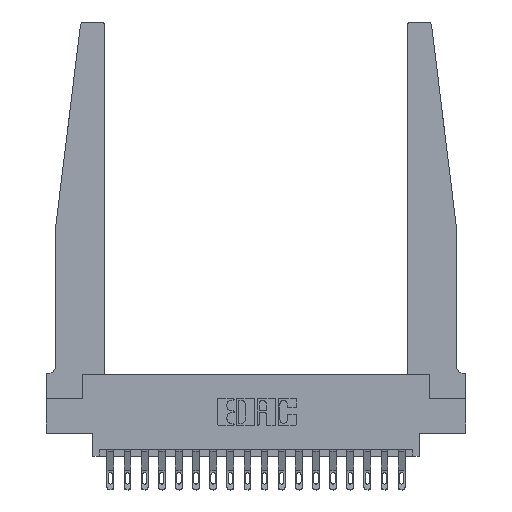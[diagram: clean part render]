
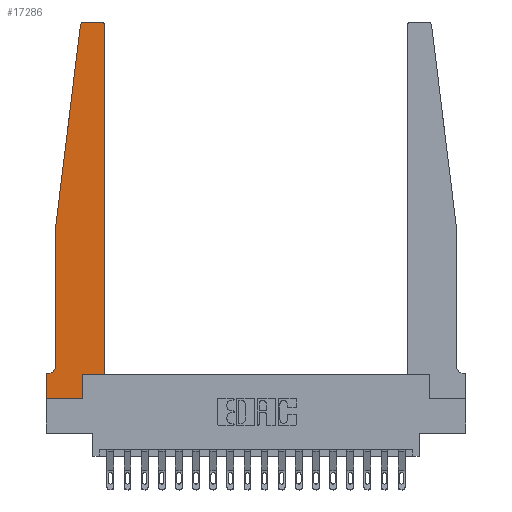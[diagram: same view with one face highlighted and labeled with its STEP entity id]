
A CAD part, top view. The second image highlights one B-rep face of the part: STEP entity #17286.
In plain terms, the highlighted planar face has unit normal (0, 0, 1).
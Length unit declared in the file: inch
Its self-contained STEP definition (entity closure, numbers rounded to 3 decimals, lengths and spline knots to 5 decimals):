
#2 = VERTEX_POINT ( 'NONE', #19551 ) ;
#553 = ORIENTED_EDGE ( 'NONE', *, *, #11119, .T. ) ;
#684 = DIRECTION ( 'NONE',  ( 0., -1., 0. ) ) ;
#895 = AXIS2_PLACEMENT_3D ( 'NONE', #1896, #1789, #16305 ) ;
#1355 = EDGE_CURVE ( 'NONE', #20141, #3529, #2249, .T. ) ;
#1683 = CARTESIAN_POINT ( 'NONE',  ( 0.425, 2.72, 0.37 ) ) ;
#1789 = DIRECTION ( 'NONE',  ( 0., 0., 1. ) ) ;
#1841 = CARTESIAN_POINT ( 'NONE',  ( 0., 0., 0.37 ) ) ;
#1896 = CARTESIAN_POINT ( 'NONE',  ( 0.27653, 2.72, 0.37 ) ) ;
#2063 = AXIS2_PLACEMENT_3D ( 'NONE', #4979, #17769, #14575 ) ;
#2169 = EDGE_CURVE ( 'NONE', #12813, #15977, #9680, .T. ) ;
#2173 = ORIENTED_EDGE ( 'NONE', *, *, #13621, .T. ) ;
#2249 = LINE ( 'NONE', #2551, #11891 ) ;
#2299 = DIRECTION ( 'NONE',  ( 0., 0., 1. ) ) ;
#2399 = PLANE ( 'NONE',  #10535 ) ;
#2513 = LINE ( 'NONE', #10821, #17166 ) ;
#2551 = CARTESIAN_POINT ( 'NONE',  ( 0.25, 2.75, 0.37 ) ) ;
#2930 = EDGE_CURVE ( 'NONE', #18368, #2, #6071, .T. ) ;
#3075 = CARTESIAN_POINT ( 'NONE',  ( 0.425, 0.18, 0.37 ) ) ;
#3437 = LINE ( 'NONE', #9772, #3441 ) ;
#3441 = VECTOR ( 'NONE', #4880, 39.37008 ) ;
#3484 = CIRCLE ( 'NONE', #8806, 0.03 ) ;
#3529 = VERTEX_POINT ( 'NONE', #12306 ) ;
#3726 = EDGE_CURVE ( 'NONE', #3529, #18368, #4199, .T. ) ;
#3802 = VECTOR ( 'NONE', #8134, 39.37008 ) ;
#4090 = LINE ( 'NONE', #15256, #7790 ) ;
#4199 = CIRCLE ( 'NONE', #895, 0.03 ) ;
#4679 = EDGE_CURVE ( 'NONE', #2, #12813, #15045, .T. ) ;
#4801 = CARTESIAN_POINT ( 'NONE',  ( 0.395, 2.72, 0.37 ) ) ;
#4880 = DIRECTION ( 'NONE',  ( 0., 1., 0. ) ) ;
#4979 = CARTESIAN_POINT ( 'NONE',  ( 0.015, 0.2375, 0.37 ) ) ;
#5279 = ORIENTED_EDGE ( 'NONE', *, *, #3726, .T. ) ;
#5497 = VECTOR ( 'NONE', #16469, 39.37008 ) ;
#5739 = ORIENTED_EDGE ( 'NONE', *, *, #15203, .T. ) ;
#6071 = LINE ( 'NONE', #15597, #6728 ) ;
#6651 = ORIENTED_EDGE ( 'NONE', *, *, #1355, .T. ) ;
#6728 = VECTOR ( 'NONE', #17109, 39.37008 ) ;
#7090 = DIRECTION ( 'NONE',  ( 0., -1., 0. ) ) ;
#7157 = VERTEX_POINT ( 'NONE', #3075 ) ;
#7790 = VECTOR ( 'NONE', #684, 39.37008 ) ;
#7908 = CARTESIAN_POINT ( 'NONE',  ( 0.2605, 0.18, 0.37 ) ) ;
#8134 = DIRECTION ( 'NONE',  ( 1., 0., 0. ) ) ;
#8539 = EDGE_CURVE ( 'NONE', #17967, #7157, #18100, .T. ) ;
#8806 = AXIS2_PLACEMENT_3D ( 'NONE', #4801, #11179, #14729 ) ;
#8868 = CARTESIAN_POINT ( 'NONE',  ( 0.065, 1.25, 0.37 ) ) ;
#9676 = ORIENTED_EDGE ( 'NONE', *, *, #12743, .T. ) ;
#9680 = CIRCLE ( 'NONE', #2063, 0.05 ) ;
#9718 = LINE ( 'NONE', #1841, #3802 ) ;
#9722 = LINE ( 'NONE', #13184, #5497 ) ;
#9772 = CARTESIAN_POINT ( 'NONE',  ( 0.425, 0.18, 0.37 ) ) ;
#9969 = CARTESIAN_POINT ( 'NONE',  ( 0.425, 0.18, 0.37 ) ) ;
#10384 = ORIENTED_EDGE ( 'NONE', *, *, #4679, .T. ) ;
#10422 = VERTEX_POINT ( 'NONE', #19532 ) ;
#10535 = AXIS2_PLACEMENT_3D ( 'NONE', #14794, #2299, #18094 ) ;
#10583 = CARTESIAN_POINT ( 'NONE',  ( 0.015, 0.1875, 0.37 ) ) ;
#10821 = CARTESIAN_POINT ( 'NONE',  ( 0.065, 0.1875, 0.37 ) ) ;
#11119 = EDGE_CURVE ( 'NONE', #7157, #15800, #3437, .T. ) ;
#11179 = DIRECTION ( 'NONE',  ( 0., 0., 1. ) ) ;
#11444 = EDGE_CURVE ( 'NONE', #15977, #19317, #2513, .T. ) ;
#11891 = VECTOR ( 'NONE', #18255, 39.37008 ) ;
#12287 = EDGE_CURVE ( 'NONE', #10422, #19627, #9718, .T. ) ;
#12306 = CARTESIAN_POINT ( 'NONE',  ( 0.27653, 2.75, 0.37 ) ) ;
#12677 = ORIENTED_EDGE ( 'NONE', *, *, #8539, .T. ) ;
#12743 = EDGE_CURVE ( 'NONE', #15800, #20141, #3484, .T. ) ;
#12771 = ORIENTED_EDGE ( 'NONE', *, *, #12287, .T. ) ;
#12813 = VERTEX_POINT ( 'NONE', #13149 ) ;
#13149 = CARTESIAN_POINT ( 'NONE',  ( 0.065, 0.2375, 0.37 ) ) ;
#13184 = CARTESIAN_POINT ( 'NONE',  ( 0.2605, 0.18, 0.37 ) ) ;
#13315 = ORIENTED_EDGE ( 'NONE', *, *, #2930, .T. ) ;
#13411 = EDGE_LOOP ( 'NONE', ( #6651, #5279, #13315, #10384, #14234, #14661, #5739, #12771, #2173, #12677, #553, #9676 ) ) ;
#13621 = EDGE_CURVE ( 'NONE', #19627, #17967, #9722, .T. ) ;
#13642 = VECTOR ( 'NONE', #7090, 39.37008 ) ;
#13999 = VECTOR ( 'NONE', #17881, 39.37008 ) ;
#14234 = ORIENTED_EDGE ( 'NONE', *, *, #2169, .T. ) ;
#14575 = DIRECTION ( 'NONE',  ( -1., 0., 0. ) ) ;
#14578 = CARTESIAN_POINT ( 'NONE',  ( 0.24675, 2.72367, 0.37 ) ) ;
#14661 = ORIENTED_EDGE ( 'NONE', *, *, #11444, .T. ) ;
#14729 = DIRECTION ( 'NONE',  ( 1., 0., 0. ) ) ;
#14794 = CARTESIAN_POINT ( 'NONE',  ( 0., 0.1875, 0.37 ) ) ;
#15045 = LINE ( 'NONE', #8868, #13642 ) ;
#15203 = EDGE_CURVE ( 'NONE', #19317, #10422, #4090, .T. ) ;
#15256 = CARTESIAN_POINT ( 'NONE',  ( 0., 0., 0.37 ) ) ;
#15597 = CARTESIAN_POINT ( 'NONE',  ( 0.065, 1.25, 0.37 ) ) ;
#15800 = VERTEX_POINT ( 'NONE', #1683 ) ;
#15977 = VERTEX_POINT ( 'NONE', #10583 ) ;
#16305 = DIRECTION ( 'NONE',  ( 1., 0., 0. ) ) ;
#16469 = DIRECTION ( 'NONE',  ( 0., 1., 0. ) ) ;
#16587 = CARTESIAN_POINT ( 'NONE',  ( 0.2605, 0., 0.37 ) ) ;
#17052 = DIRECTION ( 'NONE',  ( -1., 0., 0. ) ) ;
#17109 = DIRECTION ( 'NONE',  ( -0.122, -0.992, 0. ) ) ;
#17166 = VECTOR ( 'NONE', #17052, 39.37008 ) ;
#17286 = ADVANCED_FACE ( 'NONE', ( #20077 ), #2399, .T. ) ;
#17769 = DIRECTION ( 'NONE',  ( 0., 0., -1. ) ) ;
#17881 = DIRECTION ( 'NONE',  ( 1., 0., 0. ) ) ;
#17967 = VERTEX_POINT ( 'NONE', #7908 ) ;
#18094 = DIRECTION ( 'NONE',  ( 1., 0., 0. ) ) ;
#18100 = LINE ( 'NONE', #9969, #13999 ) ;
#18255 = DIRECTION ( 'NONE',  ( -1., 0., 0. ) ) ;
#18368 = VERTEX_POINT ( 'NONE', #14578 ) ;
#19317 = VERTEX_POINT ( 'NONE', #19922 ) ;
#19532 = CARTESIAN_POINT ( 'NONE',  ( 0., 0., 0.37 ) ) ;
#19551 = CARTESIAN_POINT ( 'NONE',  ( 0.065, 1.25, 0.37 ) ) ;
#19627 = VERTEX_POINT ( 'NONE', #16587 ) ;
#19922 = CARTESIAN_POINT ( 'NONE',  ( 0., 0.1875, 0.37 ) ) ;
#20077 = FACE_OUTER_BOUND ( 'NONE', #13411, .T. ) ;
#20141 = VERTEX_POINT ( 'NONE', #20342 ) ;
#20342 = CARTESIAN_POINT ( 'NONE',  ( 0.395, 2.75, 0.37 ) ) ;
